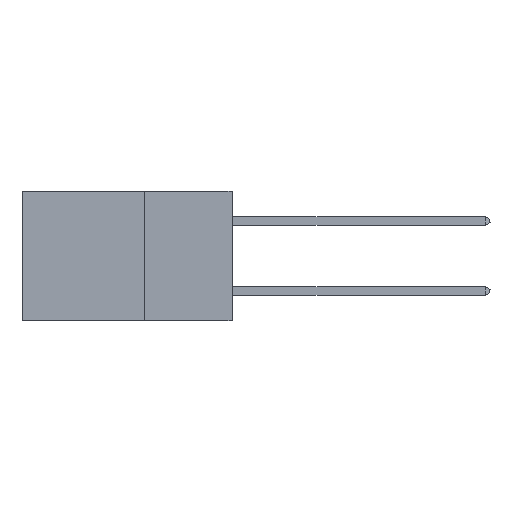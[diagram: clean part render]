
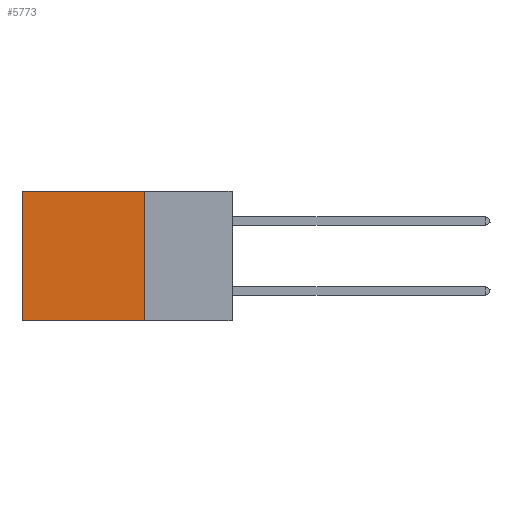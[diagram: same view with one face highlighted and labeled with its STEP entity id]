
A CAD part, left-side view. The second image highlights one B-rep face of the part: STEP entity #5773.
In plain terms, the highlighted planar face has unit normal (-1, 0, 0).
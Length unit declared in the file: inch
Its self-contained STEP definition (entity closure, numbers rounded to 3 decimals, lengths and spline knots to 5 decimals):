
#251 = CARTESIAN_POINT ( 'NONE',  ( 0.2875, 0.25, -0.37 ) ) ;
#5773 = ADVANCED_FACE ( 'NONE', ( #15494 ), #25375, .F. ) ;
#7029 = DIRECTION ( 'NONE',  ( 0., 0., -1. ) ) ;
#7835 = VECTOR ( 'NONE', #46102, 39.37008 ) ;
#9989 = ORIENTED_EDGE ( 'NONE', *, *, #13122, .F. ) ;
#13122 = EDGE_CURVE ( 'NONE', #28366, #42951, #19198, .T. ) ;
#15494 = FACE_OUTER_BOUND ( 'NONE', #20041, .T. ) ;
#15953 = EDGE_CURVE ( 'NONE', #28366, #31778, #33805, .T. ) ;
#16541 = CARTESIAN_POINT ( 'NONE',  ( 0.2875, 0.25, 0. ) ) ;
#18004 = CARTESIAN_POINT ( 'NONE',  ( 0.2875, 0.25, 0. ) ) ;
#19086 = LINE ( 'NONE', #251, #25999 ) ;
#19198 = LINE ( 'NONE', #16541, #7835 ) ;
#20041 = EDGE_LOOP ( 'NONE', ( #40748, #22559, #9989, #46447 ) ) ;
#21770 = DIRECTION ( 'NONE',  ( 0., 1., 0. ) ) ;
#21889 = CARTESIAN_POINT ( 'NONE',  ( 0.2875, 0.6, 0. ) ) ;
#22118 = CARTESIAN_POINT ( 'NONE',  ( 0.2875, 0.25, -0.37 ) ) ;
#22559 = ORIENTED_EDGE ( 'NONE', *, *, #46689, .F. ) ;
#24373 = CARTESIAN_POINT ( 'NONE',  ( 0.2875, 0.6, 0. ) ) ;
#25059 = CARTESIAN_POINT ( 'NONE',  ( 0.2875, 0.25, 0. ) ) ;
#25375 = PLANE ( 'NONE',  #27023 ) ;
#25999 = VECTOR ( 'NONE', #21770, 39.37008 ) ;
#27023 = AXIS2_PLACEMENT_3D ( 'NONE', #25059, #36065, #7029 ) ;
#27282 = LINE ( 'NONE', #24373, #41536 ) ;
#27922 = DIRECTION ( 'NONE',  ( 0., 0., -1. ) ) ;
#28366 = VERTEX_POINT ( 'NONE', #18004 ) ;
#28658 = DIRECTION ( 'NONE',  ( 0., 1., 0. ) ) ;
#31778 = VERTEX_POINT ( 'NONE', #21889 ) ;
#33805 = LINE ( 'NONE', #46854, #36092 ) ;
#36065 = DIRECTION ( 'NONE',  ( 1., 0., 0. ) ) ;
#36092 = VECTOR ( 'NONE', #28658, 39.37008 ) ;
#37090 = EDGE_CURVE ( 'NONE', #31778, #43559, #27282, .T. ) ;
#40748 = ORIENTED_EDGE ( 'NONE', *, *, #37090, .T. ) ;
#41536 = VECTOR ( 'NONE', #27922, 39.37008 ) ;
#42951 = VERTEX_POINT ( 'NONE', #22118 ) ;
#43559 = VERTEX_POINT ( 'NONE', #43972 ) ;
#43972 = CARTESIAN_POINT ( 'NONE',  ( 0.2875, 0.6, -0.37 ) ) ;
#46102 = DIRECTION ( 'NONE',  ( 0., 0., -1. ) ) ;
#46447 = ORIENTED_EDGE ( 'NONE', *, *, #15953, .T. ) ;
#46689 = EDGE_CURVE ( 'NONE', #42951, #43559, #19086, .T. ) ;
#46854 = CARTESIAN_POINT ( 'NONE',  ( 0.2875, 0.25, 0. ) ) ;
